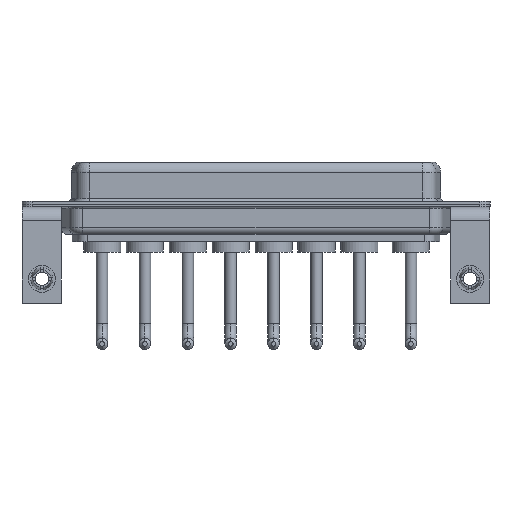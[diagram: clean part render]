
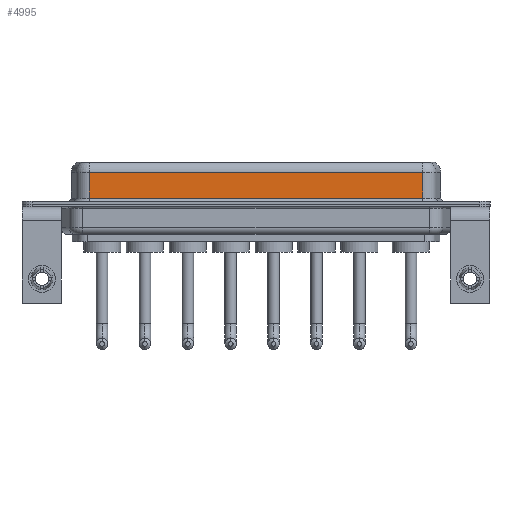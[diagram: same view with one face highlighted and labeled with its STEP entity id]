
A CAD part, front view. The second image highlights one B-rep face of the part: STEP entity #4995.
In plain terms, the highlighted planar face has unit normal (0, -1, 0).
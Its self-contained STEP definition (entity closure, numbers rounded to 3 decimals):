
#272 = EDGE_CURVE ( 'NONE', #4239, #2364, #646, .T. ) ;
#646 = LINE ( 'NONE', #2943, #9512 ) ;
#1119 = LINE ( 'NONE', #7230, #1450 ) ;
#1178 = CARTESIAN_POINT ( 'NONE',  ( 56.462, -3.95, 4.65 ) ) ;
#1450 = VECTOR ( 'NONE', #3426, 1000. ) ;
#2002 = VECTOR ( 'NONE', #5842, 1000. ) ;
#2364 = VERTEX_POINT ( 'NONE', #5878 ) ;
#2943 = CARTESIAN_POINT ( 'NONE',  ( 7.038, -3.95, 6.4 ) ) ;
#3426 = DIRECTION ( 'NONE',  ( 1., 0., 0. ) ) ;
#3548 = ORIENTED_EDGE ( 'NONE', *, *, #7165, .F. ) ;
#3562 = FACE_OUTER_BOUND ( 'NONE', #15255, .T. ) ;
#3680 = DIRECTION ( 'NONE',  ( 0., 0., -1. ) ) ;
#4239 = VERTEX_POINT ( 'NONE', #8382 ) ;
#4407 = CARTESIAN_POINT ( 'NONE',  ( 56.462, -3.95, 4.65 ) ) ;
#4995 = ADVANCED_FACE ( 'NONE', ( #3562 ), #8330, .F. ) ;
#5842 = DIRECTION ( 'NONE',  ( -1., 0., 0. ) ) ;
#5878 = CARTESIAN_POINT ( 'NONE',  ( 7.038, -3.95, 0.9 ) ) ;
#5978 = VECTOR ( 'NONE', #3680, 1000. ) ;
#6722 = ORIENTED_EDGE ( 'NONE', *, *, #272, .T. ) ;
#6939 = VERTEX_POINT ( 'NONE', #1178 ) ;
#7165 = EDGE_CURVE ( 'NONE', #6939, #7266, #9482, .T. ) ;
#7230 = CARTESIAN_POINT ( 'NONE',  ( 56.462, -3.95, 0.9 ) ) ;
#7266 = VERTEX_POINT ( 'NONE', #14693 ) ;
#7307 = ORIENTED_EDGE ( 'NONE', *, *, #10329, .T. ) ;
#7949 = DIRECTION ( 'NONE',  ( 0., 0., -1. ) ) ;
#8330 = PLANE ( 'NONE',  #14528 ) ;
#8374 = CARTESIAN_POINT ( 'NONE',  ( 56.462, -3.95, 6.4 ) ) ;
#8382 = CARTESIAN_POINT ( 'NONE',  ( 7.038, -3.95, 4.65 ) ) ;
#8931 = EDGE_CURVE ( 'NONE', #2364, #7266, #1119, .T. ) ;
#9482 = LINE ( 'NONE', #8374, #5978 ) ;
#9512 = VECTOR ( 'NONE', #7949, 1000. ) ;
#10329 = EDGE_CURVE ( 'NONE', #6939, #4239, #10594, .T. ) ;
#10594 = LINE ( 'NONE', #4407, #2002 ) ;
#10863 = CARTESIAN_POINT ( 'NONE',  ( 56.462, -3.95, 6.4 ) ) ;
#11808 = DIRECTION ( 'NONE',  ( 0., 1., 0. ) ) ;
#11964 = DIRECTION ( 'NONE',  ( 0., 0., 1. ) ) ;
#14177 = ORIENTED_EDGE ( 'NONE', *, *, #8931, .T. ) ;
#14528 = AXIS2_PLACEMENT_3D ( 'NONE', #10863, #11808, #11964 ) ;
#14693 = CARTESIAN_POINT ( 'NONE',  ( 56.462, -3.95, 0.9 ) ) ;
#15255 = EDGE_LOOP ( 'NONE', ( #3548, #7307, #6722, #14177 ) ) ;
